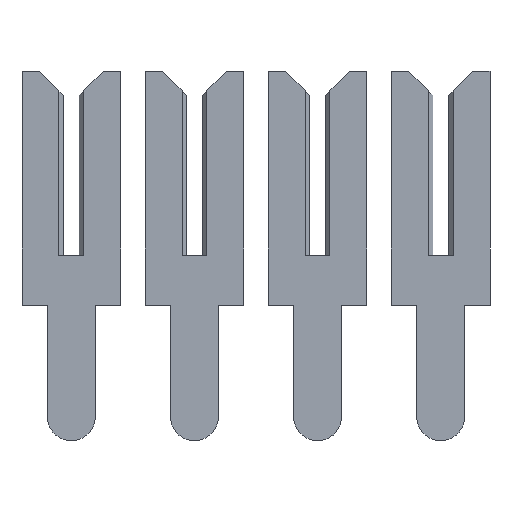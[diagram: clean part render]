
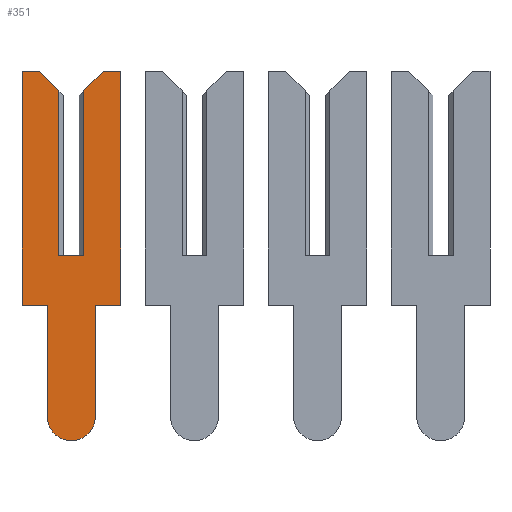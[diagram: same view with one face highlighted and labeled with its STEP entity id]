
A CAD part, top view. The second image highlights one B-rep face of the part: STEP entity #351.
In plain terms, the highlighted face is planar.
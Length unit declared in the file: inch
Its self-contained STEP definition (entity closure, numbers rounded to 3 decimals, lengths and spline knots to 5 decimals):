
#2 = EDGE_CURVE ( 'NONE', #561, #281, #409, .T. ) ;
#6 = CARTESIAN_POINT ( 'NONE',  ( -0.01, 0.15, -0.026 ) ) ;
#25 = VECTOR ( 'NONE', #417, 39.37008 ) ;
#33 = VERTEX_POINT ( 'NONE', #803 ) ;
#34 = EDGE_CURVE ( 'NONE', #281, #527, #137, .T. ) ;
#38 = LINE ( 'NONE', #565, #551 ) ;
#48 = ORIENTED_EDGE ( 'NONE', *, *, #2, .F. ) ;
#68 = EDGE_CURVE ( 'NONE', #344, #398, #97, .T. ) ;
#87 = LINE ( 'NONE', #285, #872 ) ;
#97 = LINE ( 'NONE', #6, #373 ) ;
#104 = DIRECTION ( 'NONE',  ( 0., -1., 0. ) ) ;
#117 = EDGE_CURVE ( 'NONE', #739, #592, #647, .T. ) ;
#130 = CARTESIAN_POINT ( 'NONE',  ( -0.01, -0.1305, 0.0195 ) ) ;
#135 = AXIS2_PLACEMENT_3D ( 'NONE', #520, #365, #446 ) ;
#137 = LINE ( 'NONE', #368, #688 ) ;
#143 = ORIENTED_EDGE ( 'NONE', *, *, #146, .F. ) ;
#146 = EDGE_CURVE ( 'NONE', #601, #561, #816, .T. ) ;
#162 = DIRECTION ( 'NONE',  ( 0., -1., 0. ) ) ;
#172 = EDGE_CURVE ( 'NONE', #182, #601, #385, .T. ) ;
#175 = VECTOR ( 'NONE', #780, 39.37008 ) ;
#176 = PLANE ( 'NONE',  #876 ) ;
#181 = VECTOR ( 'NONE', #104, 39.37008 ) ;
#182 = VERTEX_POINT ( 'NONE', #815 ) ;
#186 = CARTESIAN_POINT ( 'NONE',  ( -0.01, -0.1305, 0. ) ) ;
#197 = CARTESIAN_POINT ( 'NONE',  ( -0.01, 0., 0.0065 ) ) ;
#239 = CARTESIAN_POINT ( 'NONE',  ( -0.01, -0.04, 0.04 ) ) ;
#241 = CARTESIAN_POINT ( 'NONE',  ( -0.01, 0.15, -0.04 ) ) ;
#256 = CARTESIAN_POINT ( 'NONE',  ( -0.01, 0.15, 0.04 ) ) ;
#258 = ORIENTED_EDGE ( 'NONE', *, *, #117, .F. ) ;
#267 = EDGE_CURVE ( 'NONE', #804, #377, #316, .T. ) ;
#274 = CARTESIAN_POINT ( 'NONE',  ( -0.01, 0.1305, -0.0065 ) ) ;
#281 = VERTEX_POINT ( 'NONE', #680 ) ;
#284 = LINE ( 'NONE', #274, #795 ) ;
#285 = CARTESIAN_POINT ( 'NONE',  ( -0.01, 0.1305, 0.0065 ) ) ;
#304 = EDGE_LOOP ( 'NONE', ( #837, #826, #258, #764, #503, #432, #402, #671, #48, #143, #861, #459, #817, #439 ) ) ;
#316 = LINE ( 'NONE', #318, #869 ) ;
#318 = CARTESIAN_POINT ( 'NONE',  ( -0.01, 0.15, 0.01 ) ) ;
#336 = CARTESIAN_POINT ( 'NONE',  ( -0.01, -0.04, 0.0195 ) ) ;
#344 = VERTEX_POINT ( 'NONE', #241 ) ;
#351 = ADVANCED_FACE ( 'NONE', ( #537 ), #176, .F. ) ;
#353 = EDGE_CURVE ( 'NONE', #792, #896, #576, .T. ) ;
#365 = DIRECTION ( 'NONE',  ( 1., 0., 0. ) ) ;
#368 = CARTESIAN_POINT ( 'NONE',  ( -0.01, -0.04, -0.0195 ) ) ;
#372 = CARTESIAN_POINT ( 'NONE',  ( -0.01, 0.134, 0.01 ) ) ;
#373 = VECTOR ( 'NONE', #578, 39.37008 ) ;
#377 = VERTEX_POINT ( 'NONE', #757 ) ;
#385 = LINE ( 'NONE', #239, #860 ) ;
#393 = DIRECTION ( 'NONE',  ( 1., 0., 0. ) ) ;
#398 = VERTEX_POINT ( 'NONE', #900 ) ;
#402 = ORIENTED_EDGE ( 'NONE', *, *, #420, .F. ) ;
#407 = DIRECTION ( 'NONE',  ( 0., -0.707, 0.707 ) ) ;
#409 = CIRCLE ( 'NONE', #135, 0.0195 ) ;
#417 = DIRECTION ( 'NONE',  ( 0., -1., 0. ) ) ;
#420 = EDGE_CURVE ( 'NONE', #527, #33, #473, .T. ) ;
#432 = ORIENTED_EDGE ( 'NONE', *, *, #617, .F. ) ;
#439 = ORIENTED_EDGE ( 'NONE', *, *, #818, .F. ) ;
#446 = DIRECTION ( 'NONE',  ( 0., 0., -1. ) ) ;
#455 = VECTOR ( 'NONE', #162, 39.37008 ) ;
#459 = ORIENTED_EDGE ( 'NONE', *, *, #632, .F. ) ;
#467 = DIRECTION ( 'NONE',  ( 0., 0., 1. ) ) ;
#471 = CARTESIAN_POINT ( 'NONE',  ( -0.01, 0.15, 0.026 ) ) ;
#473 = LINE ( 'NONE', #609, #642 ) ;
#499 = VECTOR ( 'NONE', #467, 39.37008 ) ;
#503 = ORIENTED_EDGE ( 'NONE', *, *, #68, .F. ) ;
#511 = DIRECTION ( 'NONE',  ( 0., 1., 0. ) ) ;
#520 = CARTESIAN_POINT ( 'NONE',  ( -0.01, -0.1305, 0. ) ) ;
#527 = VERTEX_POINT ( 'NONE', #554 ) ;
#533 = EDGE_CURVE ( 'NONE', #592, #377, #808, .T. ) ;
#536 = DIRECTION ( 'NONE',  ( 0., 0., -1. ) ) ;
#537 = FACE_OUTER_BOUND ( 'NONE', #304, .T. ) ;
#551 = VECTOR ( 'NONE', #843, 39.37008 ) ;
#554 = CARTESIAN_POINT ( 'NONE',  ( -0.01, -0.04, -0.0195 ) ) ;
#561 = VERTEX_POINT ( 'NONE', #130 ) ;
#565 = CARTESIAN_POINT ( 'NONE',  ( -0.01, 0.15, -0.04 ) ) ;
#576 = LINE ( 'NONE', #471, #499 ) ;
#578 = DIRECTION ( 'NONE',  ( 0., 0., 1. ) ) ;
#588 = DIRECTION ( 'NONE',  ( 0., 0.707, 0.707 ) ) ;
#592 = VERTEX_POINT ( 'NONE', #626 ) ;
#601 = VERTEX_POINT ( 'NONE', #336 ) ;
#602 = DIRECTION ( 'NONE',  ( 0., 0., -1. ) ) ;
#609 = CARTESIAN_POINT ( 'NONE',  ( -0.01, -0.04, -0.04 ) ) ;
#616 = DIRECTION ( 'NONE',  ( 0., 0., -1. ) ) ;
#617 = EDGE_CURVE ( 'NONE', #33, #344, #38, .T. ) ;
#626 = CARTESIAN_POINT ( 'NONE',  ( -0.01, 0., -0.01 ) ) ;
#632 = EDGE_CURVE ( 'NONE', #896, #182, #644, .T. ) ;
#642 = VECTOR ( 'NONE', #536, 39.37008 ) ;
#644 = LINE ( 'NONE', #256, #25 ) ;
#647 = LINE ( 'NONE', #864, #455 ) ;
#658 = CARTESIAN_POINT ( 'NONE',  ( -0.01, 0.134, -0.01 ) ) ;
#671 = ORIENTED_EDGE ( 'NONE', *, *, #34, .F. ) ;
#680 = CARTESIAN_POINT ( 'NONE',  ( -0.01, -0.1305, -0.0195 ) ) ;
#688 = VECTOR ( 'NONE', #511, 39.37008 ) ;
#689 = EDGE_CURVE ( 'NONE', #398, #739, #284, .T. ) ;
#719 = CARTESIAN_POINT ( 'NONE',  ( -0.01, 0.15, 0.026 ) ) ;
#735 = CARTESIAN_POINT ( 'NONE',  ( -0.01, -0.04, 0.0195 ) ) ;
#739 = VERTEX_POINT ( 'NONE', #658 ) ;
#757 = CARTESIAN_POINT ( 'NONE',  ( -0.01, 0., 0.01 ) ) ;
#764 = ORIENTED_EDGE ( 'NONE', *, *, #689, .F. ) ;
#780 = DIRECTION ( 'NONE',  ( 0., 0., 1. ) ) ;
#792 = VERTEX_POINT ( 'NONE', #719 ) ;
#795 = VECTOR ( 'NONE', #407, 39.37008 ) ;
#803 = CARTESIAN_POINT ( 'NONE',  ( -0.01, -0.04, -0.04 ) ) ;
#804 = VERTEX_POINT ( 'NONE', #372 ) ;
#808 = LINE ( 'NONE', #197, #175 ) ;
#809 = CARTESIAN_POINT ( 'NONE',  ( -0.01, 0.15, 0.04 ) ) ;
#815 = CARTESIAN_POINT ( 'NONE',  ( -0.01, -0.04, 0.04 ) ) ;
#816 = LINE ( 'NONE', #735, #181 ) ;
#817 = ORIENTED_EDGE ( 'NONE', *, *, #353, .F. ) ;
#818 = EDGE_CURVE ( 'NONE', #804, #792, #87, .T. ) ;
#823 = DIRECTION ( 'NONE',  ( 0., -1., 0. ) ) ;
#826 = ORIENTED_EDGE ( 'NONE', *, *, #533, .F. ) ;
#837 = ORIENTED_EDGE ( 'NONE', *, *, #267, .T. ) ;
#843 = DIRECTION ( 'NONE',  ( 0., 1., 0. ) ) ;
#860 = VECTOR ( 'NONE', #602, 39.37008 ) ;
#861 = ORIENTED_EDGE ( 'NONE', *, *, #172, .F. ) ;
#864 = CARTESIAN_POINT ( 'NONE',  ( -0.01, -0.1305, -0.01 ) ) ;
#869 = VECTOR ( 'NONE', #823, 39.37008 ) ;
#872 = VECTOR ( 'NONE', #588, 39.37008 ) ;
#876 = AXIS2_PLACEMENT_3D ( 'NONE', #186, #393, #616 ) ;
#896 = VERTEX_POINT ( 'NONE', #809 ) ;
#900 = CARTESIAN_POINT ( 'NONE',  ( -0.01, 0.15, -0.026 ) ) ;
